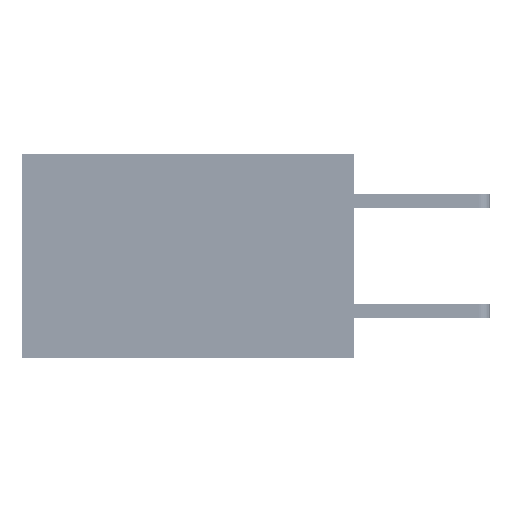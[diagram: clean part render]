
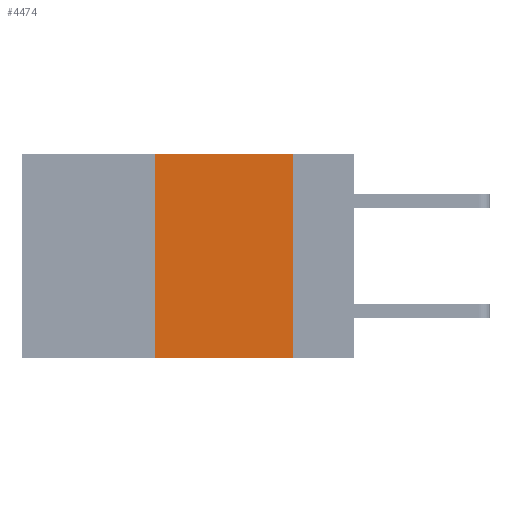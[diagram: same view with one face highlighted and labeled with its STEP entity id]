
A CAD part, left-side view. The second image highlights one B-rep face of the part: STEP entity #4474.
In plain terms, the highlighted planar face has unit normal (-1, 0, 0).
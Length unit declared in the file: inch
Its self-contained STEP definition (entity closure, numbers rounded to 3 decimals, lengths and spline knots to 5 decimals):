
#209 = CARTESIAN_POINT ( 'NONE',  ( 0., 0.36, 0. ) ) ;
#1225 = DIRECTION ( 'NONE',  ( 0., -1., 0. ) ) ;
#1732 = CARTESIAN_POINT ( 'NONE',  ( 0., 0.11, -0.37 ) ) ;
#4474 = ADVANCED_FACE ( 'NONE', ( #42921 ), #23595, .F. ) ;
#5438 = LINE ( 'NONE', #9644, #17809 ) ;
#6046 = VECTOR ( 'NONE', #37271, 39.37008 ) ;
#6063 = EDGE_CURVE ( 'NONE', #41327, #33126, #11786, .T. ) ;
#6377 = VERTEX_POINT ( 'NONE', #1732 ) ;
#6921 = CARTESIAN_POINT ( 'NONE',  ( 0., 0.36, -0.37 ) ) ;
#7933 = VECTOR ( 'NONE', #1225, 39.37008 ) ;
#9080 = LINE ( 'NONE', #37100, #7933 ) ;
#9122 = AXIS2_PLACEMENT_3D ( 'NONE', #30856, #16503, #16040 ) ;
#9491 = DIRECTION ( 'NONE',  ( 0., -1., 0. ) ) ;
#9644 = CARTESIAN_POINT ( 'NONE',  ( 0., 0.6, 0. ) ) ;
#10335 = EDGE_CURVE ( 'NONE', #33126, #32906, #5438, .T. ) ;
#11786 = LINE ( 'NONE', #209, #25902 ) ;
#12010 = EDGE_LOOP ( 'NONE', ( #14777, #38621, #26660, #23878 ) ) ;
#14777 = ORIENTED_EDGE ( 'NONE', *, *, #43891, .F. ) ;
#14814 = CARTESIAN_POINT ( 'NONE',  ( 0., 0.36, 0. ) ) ;
#16040 = DIRECTION ( 'NONE',  ( 0., 0., -1. ) ) ;
#16503 = DIRECTION ( 'NONE',  ( 1., 0., 0. ) ) ;
#17527 = CARTESIAN_POINT ( 'NONE',  ( 0., 0.11, 0. ) ) ;
#17809 = VECTOR ( 'NONE', #9491, 39.37008 ) ;
#19582 = EDGE_CURVE ( 'NONE', #41327, #6377, #9080, .T. ) ;
#23595 = PLANE ( 'NONE',  #9122 ) ;
#23878 = ORIENTED_EDGE ( 'NONE', *, *, #19582, .T. ) ;
#25902 = VECTOR ( 'NONE', #35905, 39.37008 ) ;
#26660 = ORIENTED_EDGE ( 'NONE', *, *, #6063, .F. ) ;
#30856 = CARTESIAN_POINT ( 'NONE',  ( 0., 0.6, 0. ) ) ;
#32906 = VERTEX_POINT ( 'NONE', #17527 ) ;
#33126 = VERTEX_POINT ( 'NONE', #14814 ) ;
#35905 = DIRECTION ( 'NONE',  ( 0., 0., 1. ) ) ;
#37100 = CARTESIAN_POINT ( 'NONE',  ( 0., 0.6, -0.37 ) ) ;
#37271 = DIRECTION ( 'NONE',  ( 0., 0., -1. ) ) ;
#38621 = ORIENTED_EDGE ( 'NONE', *, *, #10335, .F. ) ;
#40915 = LINE ( 'NONE', #44011, #6046 ) ;
#41327 = VERTEX_POINT ( 'NONE', #6921 ) ;
#42921 = FACE_OUTER_BOUND ( 'NONE', #12010, .T. ) ;
#43891 = EDGE_CURVE ( 'NONE', #32906, #6377, #40915, .T. ) ;
#44011 = CARTESIAN_POINT ( 'NONE',  ( 0., 0.11, 0. ) ) ;
